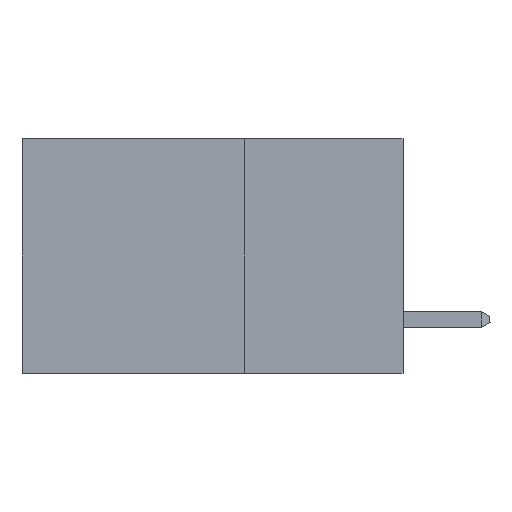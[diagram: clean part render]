
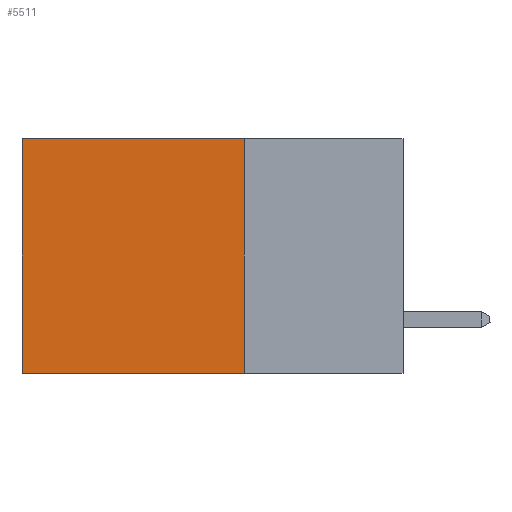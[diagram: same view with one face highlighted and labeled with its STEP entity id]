
A CAD part, left-side view. The second image highlights one B-rep face of the part: STEP entity #5511.
In plain terms, the highlighted planar face has unit normal (-1, 0, 0).
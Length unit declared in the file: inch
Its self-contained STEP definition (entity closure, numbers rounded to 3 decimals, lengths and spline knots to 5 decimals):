
#243 = EDGE_LOOP ( 'NONE', ( #14134, #15472, #5584, #17724 ) ) ;
#518 = VECTOR ( 'NONE', #9523, 39.37008 ) ;
#733 = CARTESIAN_POINT ( 'NONE',  ( 0.2875, 0.25, -0.37 ) ) ;
#1363 = VERTEX_POINT ( 'NONE', #12714 ) ;
#2880 = CARTESIAN_POINT ( 'NONE',  ( 0.2875, 0.25, 0. ) ) ;
#3145 = EDGE_CURVE ( 'NONE', #8121, #3679, #10072, .T. ) ;
#3453 = VERTEX_POINT ( 'NONE', #12162 ) ;
#3552 = CARTESIAN_POINT ( 'NONE',  ( 0.2875, 0.6, 0. ) ) ;
#3679 = VERTEX_POINT ( 'NONE', #13163 ) ;
#3760 = LINE ( 'NONE', #15911, #10997 ) ;
#4400 = AXIS2_PLACEMENT_3D ( 'NONE', #2880, #7173, #17247 ) ;
#5511 = ADVANCED_FACE ( 'NONE', ( #5848 ), #11491, .F. ) ;
#5584 = ORIENTED_EDGE ( 'NONE', *, *, #7936, .F. ) ;
#5848 = FACE_OUTER_BOUND ( 'NONE', #243, .T. ) ;
#6676 = DIRECTION ( 'NONE',  ( 0., 0., -1. ) ) ;
#7173 = DIRECTION ( 'NONE',  ( 1., 0., 0. ) ) ;
#7936 = EDGE_CURVE ( 'NONE', #1363, #3453, #3760, .T. ) ;
#8121 = VERTEX_POINT ( 'NONE', #12334 ) ;
#8629 = LINE ( 'NONE', #15557, #17634 ) ;
#9523 = DIRECTION ( 'NONE',  ( 0., 1., 0. ) ) ;
#10072 = LINE ( 'NONE', #3552, #16772 ) ;
#10889 = LINE ( 'NONE', #733, #518 ) ;
#10997 = VECTOR ( 'NONE', #6676, 39.37008 ) ;
#11200 = EDGE_CURVE ( 'NONE', #3453, #3679, #10889, .T. ) ;
#11491 = PLANE ( 'NONE',  #4400 ) ;
#12162 = CARTESIAN_POINT ( 'NONE',  ( 0.2875, 0.25, -0.37 ) ) ;
#12334 = CARTESIAN_POINT ( 'NONE',  ( 0.2875, 0.6, 0. ) ) ;
#12714 = CARTESIAN_POINT ( 'NONE',  ( 0.2875, 0.25, 0. ) ) ;
#13163 = CARTESIAN_POINT ( 'NONE',  ( 0.2875, 0.6, -0.37 ) ) ;
#13271 = EDGE_CURVE ( 'NONE', #1363, #8121, #8629, .T. ) ;
#13384 = DIRECTION ( 'NONE',  ( 0., 0., -1. ) ) ;
#14134 = ORIENTED_EDGE ( 'NONE', *, *, #3145, .T. ) ;
#14360 = DIRECTION ( 'NONE',  ( 0., 1., 0. ) ) ;
#15472 = ORIENTED_EDGE ( 'NONE', *, *, #11200, .F. ) ;
#15557 = CARTESIAN_POINT ( 'NONE',  ( 0.2875, 0.25, 0. ) ) ;
#15911 = CARTESIAN_POINT ( 'NONE',  ( 0.2875, 0.25, 0. ) ) ;
#16772 = VECTOR ( 'NONE', #13384, 39.37008 ) ;
#17247 = DIRECTION ( 'NONE',  ( 0., 0., -1. ) ) ;
#17634 = VECTOR ( 'NONE', #14360, 39.37008 ) ;
#17724 = ORIENTED_EDGE ( 'NONE', *, *, #13271, .T. ) ;
